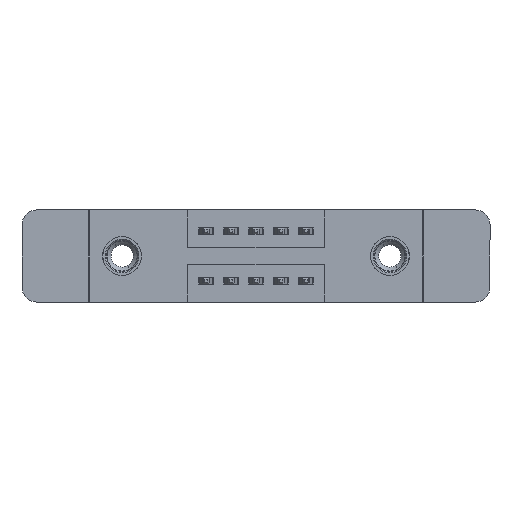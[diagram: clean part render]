
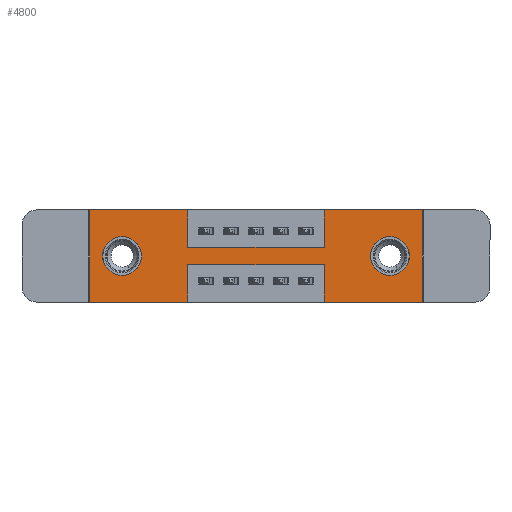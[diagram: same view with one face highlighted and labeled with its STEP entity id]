
A CAD part, front view. The second image highlights one B-rep face of the part: STEP entity #4800.
In plain terms, the highlighted planar face has unit normal (0, -1, 0).
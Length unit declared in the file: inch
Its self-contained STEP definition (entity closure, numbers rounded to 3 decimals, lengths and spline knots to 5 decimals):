
#3 = LINE ( 'NONE', #292, #5601 ) ;
#292 = CARTESIAN_POINT ( 'NONE',  ( 0., 0., -0.37 ) ) ;
#416 = EDGE_CURVE ( 'NONE', #4822, #11302, #3, .T. ) ;
#426 = CARTESIAN_POINT ( 'NONE',  ( 0.3925, 0., -0.22 ) ) ;
#496 = ORIENTED_EDGE ( 'NONE', *, *, #11588, .F. ) ;
#670 = DIRECTION ( 'NONE',  ( 0., 0., 1. ) ) ;
#716 = VECTOR ( 'NONE', #8701, 39.37008 ) ;
#907 = LINE ( 'NONE', #1181, #716 ) ;
#1010 = LINE ( 'NONE', #8750, #2874 ) ;
#1039 = DIRECTION ( 'NONE',  ( 1., 0., 0. ) ) ;
#1097 = VERTEX_POINT ( 'NONE', #7785 ) ;
#1137 = DIRECTION ( 'NONE',  ( -1., 0., 0. ) ) ;
#1166 = LINE ( 'NONE', #12586, #13623 ) ;
#1181 = CARTESIAN_POINT ( 'NONE',  ( 1.335, 0., 0. ) ) ;
#1237 = CIRCLE ( 'NONE', #2409, 0.078 ) ;
#1652 = VERTEX_POINT ( 'NONE', #9212 ) ;
#1668 = VERTEX_POINT ( 'NONE', #12426 ) ;
#1885 = DIRECTION ( 'NONE',  ( -1., 0., 0. ) ) ;
#2041 = EDGE_CURVE ( 'NONE', #1652, #6585, #8284, .T. ) ;
#2051 = EDGE_CURVE ( 'NONE', #4505, #1668, #4883, .T. ) ;
#2076 = CARTESIAN_POINT ( 'NONE',  ( 0., 0., -0.37 ) ) ;
#2092 = CARTESIAN_POINT ( 'NONE',  ( 0.3925, 0., -0.37 ) ) ;
#2102 = FACE_BOUND ( 'NONE', #9747, .T. ) ;
#2117 = VERTEX_POINT ( 'NONE', #7474 ) ;
#2208 = DIRECTION ( 'NONE',  ( 0., 0., 1. ) ) ;
#2220 = ORIENTED_EDGE ( 'NONE', *, *, #7983, .T. ) ;
#2334 = CARTESIAN_POINT ( 'NONE',  ( 0.9425, 0., -0.15 ) ) ;
#2409 = AXIS2_PLACEMENT_3D ( 'NONE', #11289, #12338, #5776 ) ;
#2537 = CARTESIAN_POINT ( 'NONE',  ( 0.9425, 0., 0. ) ) ;
#2652 = DIRECTION ( 'NONE',  ( 0., 0., -1. ) ) ;
#2795 = EDGE_CURVE ( 'NONE', #6585, #11439, #4030, .T. ) ;
#2835 = CARTESIAN_POINT ( 'NONE',  ( 0.3925, 0., -0.37 ) ) ;
#2874 = VECTOR ( 'NONE', #1137, 39.37008 ) ;
#2973 = LINE ( 'NONE', #2835, #4999 ) ;
#2982 = DIRECTION ( 'NONE',  ( 0., 1., 0. ) ) ;
#3027 = ORIENTED_EDGE ( 'NONE', *, *, #4983, .F. ) ;
#3295 = VERTEX_POINT ( 'NONE', #13199 ) ;
#3360 = VERTEX_POINT ( 'NONE', #426 ) ;
#3368 = VERTEX_POINT ( 'NONE', #12347 ) ;
#3503 = EDGE_CURVE ( 'NONE', #1668, #1652, #7586, .T. ) ;
#3528 = EDGE_CURVE ( 'NONE', #2117, #9010, #12877, .T. ) ;
#3968 = ORIENTED_EDGE ( 'NONE', *, *, #2041, .F. ) ;
#4030 = LINE ( 'NONE', #5569, #12054 ) ;
#4505 = VERTEX_POINT ( 'NONE', #7801 ) ;
#4800 = ADVANCED_FACE ( 'NONE', ( #2102, #8733, #5839 ), #9302, .T. ) ;
#4822 = VERTEX_POINT ( 'NONE', #2092 ) ;
#4883 = LINE ( 'NONE', #6361, #9656 ) ;
#4903 = CARTESIAN_POINT ( 'NONE',  ( 0.9425, 0., -0.37 ) ) ;
#4948 = ORIENTED_EDGE ( 'NONE', *, *, #8643, .T. ) ;
#4983 = EDGE_CURVE ( 'NONE', #5358, #3295, #907, .T. ) ;
#4999 = VECTOR ( 'NONE', #2652, 39.37008 ) ;
#5060 = DIRECTION ( 'NONE',  ( 0., -1., 0. ) ) ;
#5214 = AXIS2_PLACEMENT_3D ( 'NONE', #9393, #5060, #12699 ) ;
#5226 = CARTESIAN_POINT ( 'NONE',  ( 1.205, 0., -0.185 ) ) ;
#5292 = LINE ( 'NONE', #6031, #9049 ) ;
#5351 = VECTOR ( 'NONE', #5822, 39.37008 ) ;
#5358 = VERTEX_POINT ( 'NONE', #13708 ) ;
#5569 = CARTESIAN_POINT ( 'NONE',  ( 0.9425, 0., 0. ) ) ;
#5601 = VECTOR ( 'NONE', #8845, 39.37008 ) ;
#5619 = CARTESIAN_POINT ( 'NONE',  ( 0.13, 0., -0.185 ) ) ;
#5626 = AXIS2_PLACEMENT_3D ( 'NONE', #5226, #13983, #6124 ) ;
#5733 = VECTOR ( 'NONE', #9647, 39.37008 ) ;
#5776 = DIRECTION ( 'NONE',  ( 0., 0., -1. ) ) ;
#5822 = DIRECTION ( 'NONE',  ( 0., 0., 1. ) ) ;
#5839 = FACE_OUTER_BOUND ( 'NONE', #12225, .T. ) ;
#5846 = CIRCLE ( 'NONE', #13122, 0.078 ) ;
#5928 = CIRCLE ( 'NONE', #5626, 0.078 ) ;
#5963 = CARTESIAN_POINT ( 'NONE',  ( 0.9425, 0., -0.22 ) ) ;
#6031 = CARTESIAN_POINT ( 'NONE',  ( 0.3925, 0., -0.22 ) ) ;
#6124 = DIRECTION ( 'NONE',  ( 0., 0., -1. ) ) ;
#6341 = AXIS2_PLACEMENT_3D ( 'NONE', #5619, #6590, #12234 ) ;
#6361 = CARTESIAN_POINT ( 'NONE',  ( 0., 0., 0. ) ) ;
#6379 = ORIENTED_EDGE ( 'NONE', *, *, #2795, .F. ) ;
#6585 = VERTEX_POINT ( 'NONE', #2334 ) ;
#6590 = DIRECTION ( 'NONE',  ( 0., 1., 0. ) ) ;
#7081 = ORIENTED_EDGE ( 'NONE', *, *, #2051, .F. ) ;
#7271 = ORIENTED_EDGE ( 'NONE', *, *, #14020, .T. ) ;
#7446 = ORIENTED_EDGE ( 'NONE', *, *, #3528, .F. ) ;
#7474 = CARTESIAN_POINT ( 'NONE',  ( 0.9425, 0., -0.37 ) ) ;
#7586 = LINE ( 'NONE', #12481, #8595 ) ;
#7621 = EDGE_CURVE ( 'NONE', #3360, #4822, #2973, .T. ) ;
#7785 = CARTESIAN_POINT ( 'NONE',  ( 1.205, 0., -0.107 ) ) ;
#7801 = CARTESIAN_POINT ( 'NONE',  ( 0., 0., 0. ) ) ;
#7983 = EDGE_CURVE ( 'NONE', #9025, #3368, #10651, .T. ) ;
#8284 = LINE ( 'NONE', #9599, #5733 ) ;
#8595 = VECTOR ( 'NONE', #13579, 39.37008 ) ;
#8643 = EDGE_CURVE ( 'NONE', #3368, #9025, #5846, .T. ) ;
#8701 = DIRECTION ( 'NONE',  ( 0., 0., -1. ) ) ;
#8733 = FACE_BOUND ( 'NONE', #9324, .T. ) ;
#8750 = CARTESIAN_POINT ( 'NONE',  ( 0., 0., -0.37 ) ) ;
#8845 = DIRECTION ( 'NONE',  ( -1., 0., 0. ) ) ;
#9010 = VERTEX_POINT ( 'NONE', #5963 ) ;
#9025 = VERTEX_POINT ( 'NONE', #12686 ) ;
#9049 = VECTOR ( 'NONE', #1885, 39.37008 ) ;
#9212 = CARTESIAN_POINT ( 'NONE',  ( 0.3925, 0., -0.15 ) ) ;
#9302 = PLANE ( 'NONE',  #5214 ) ;
#9324 = EDGE_LOOP ( 'NONE', ( #2220, #4948 ) ) ;
#9393 = CARTESIAN_POINT ( 'NONE',  ( 0., 0., -0.37 ) ) ;
#9454 = ORIENTED_EDGE ( 'NONE', *, *, #3503, .F. ) ;
#9532 = CARTESIAN_POINT ( 'NONE',  ( 0.13, 0., -0.185 ) ) ;
#9562 = EDGE_CURVE ( 'NONE', #9010, #3360, #5292, .T. ) ;
#9573 = VECTOR ( 'NONE', #10268, 39.37008 ) ;
#9576 = ORIENTED_EDGE ( 'NONE', *, *, #11221, .F. ) ;
#9599 = CARTESIAN_POINT ( 'NONE',  ( 0.3925, 0., -0.15 ) ) ;
#9647 = DIRECTION ( 'NONE',  ( 1., 0., 0. ) ) ;
#9656 = VECTOR ( 'NONE', #1039, 39.37008 ) ;
#9747 = EDGE_LOOP ( 'NONE', ( #7271, #13981 ) ) ;
#9919 = LINE ( 'NONE', #13715, #9573 ) ;
#10081 = ORIENTED_EDGE ( 'NONE', *, *, #416, .F. ) ;
#10268 = DIRECTION ( 'NONE',  ( 1., 0., 0. ) ) ;
#10651 = CIRCLE ( 'NONE', #6341, 0.078 ) ;
#10857 = CARTESIAN_POINT ( 'NONE',  ( 1.205, 0., -0.263 ) ) ;
#11221 = EDGE_CURVE ( 'NONE', #3295, #2117, #1010, .T. ) ;
#11289 = CARTESIAN_POINT ( 'NONE',  ( 1.205, 0., -0.185 ) ) ;
#11302 = VERTEX_POINT ( 'NONE', #2076 ) ;
#11439 = VERTEX_POINT ( 'NONE', #2537 ) ;
#11588 = EDGE_CURVE ( 'NONE', #11302, #4505, #1166, .T. ) ;
#11695 = EDGE_CURVE ( 'NONE', #12411, #1097, #5928, .T. ) ;
#11707 = DIRECTION ( 'NONE',  ( 0., 0., 1. ) ) ;
#12054 = VECTOR ( 'NONE', #2208, 39.37008 ) ;
#12055 = ORIENTED_EDGE ( 'NONE', *, *, #9562, .F. ) ;
#12225 = EDGE_LOOP ( 'NONE', ( #13880, #12055, #7446, #9576, #3027, #13217, #6379, #3968, #9454, #7081, #496, #10081 ) ) ;
#12234 = DIRECTION ( 'NONE',  ( 0., 0., 1. ) ) ;
#12338 = DIRECTION ( 'NONE',  ( 0., 1., 0. ) ) ;
#12347 = CARTESIAN_POINT ( 'NONE',  ( 0.13, 0., -0.263 ) ) ;
#12411 = VERTEX_POINT ( 'NONE', #10857 ) ;
#12426 = CARTESIAN_POINT ( 'NONE',  ( 0.3925, 0., 0. ) ) ;
#12481 = CARTESIAN_POINT ( 'NONE',  ( 0.3925, 0., 0. ) ) ;
#12586 = CARTESIAN_POINT ( 'NONE',  ( 0., 0., 0. ) ) ;
#12686 = CARTESIAN_POINT ( 'NONE',  ( 0.13, 0., -0.107 ) ) ;
#12699 = DIRECTION ( 'NONE',  ( 0., 0., -1. ) ) ;
#12877 = LINE ( 'NONE', #4903, #5351 ) ;
#13122 = AXIS2_PLACEMENT_3D ( 'NONE', #9532, #2982, #11707 ) ;
#13199 = CARTESIAN_POINT ( 'NONE',  ( 1.335, 0., -0.37 ) ) ;
#13217 = ORIENTED_EDGE ( 'NONE', *, *, #14064, .F. ) ;
#13579 = DIRECTION ( 'NONE',  ( 0., 0., -1. ) ) ;
#13623 = VECTOR ( 'NONE', #670, 39.37008 ) ;
#13708 = CARTESIAN_POINT ( 'NONE',  ( 1.335, 0., 0. ) ) ;
#13715 = CARTESIAN_POINT ( 'NONE',  ( 0., 0., 0. ) ) ;
#13880 = ORIENTED_EDGE ( 'NONE', *, *, #7621, .F. ) ;
#13981 = ORIENTED_EDGE ( 'NONE', *, *, #11695, .T. ) ;
#13983 = DIRECTION ( 'NONE',  ( 0., 1., 0. ) ) ;
#14020 = EDGE_CURVE ( 'NONE', #1097, #12411, #1237, .T. ) ;
#14064 = EDGE_CURVE ( 'NONE', #11439, #5358, #9919, .T. ) ;
